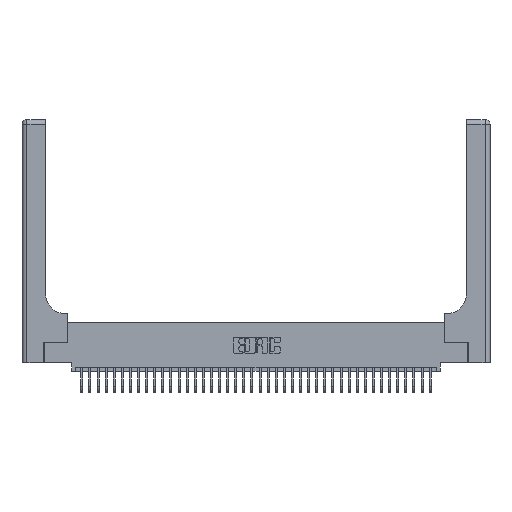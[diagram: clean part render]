
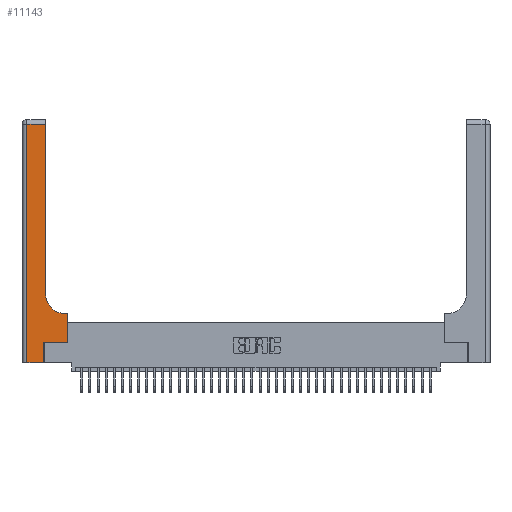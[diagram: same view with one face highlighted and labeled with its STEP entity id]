
A CAD part, top view. The second image highlights one B-rep face of the part: STEP entity #11143.
In plain terms, the highlighted planar face has unit normal (0, 0, 1).
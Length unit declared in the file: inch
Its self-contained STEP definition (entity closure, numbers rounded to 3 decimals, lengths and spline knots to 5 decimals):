
#72 = AXIS2_PLACEMENT_3D ( 'NONE', #17433, #11621, #32320 ) ;
#553 = CARTESIAN_POINT ( 'NONE',  ( 0.06, 0., 0.37 ) ) ;
#1645 = ORIENTED_EDGE ( 'NONE', *, *, #7474, .T. ) ;
#1949 = VECTOR ( 'NONE', #23740, 39.37008 ) ;
#2693 = CARTESIAN_POINT ( 'NONE',  ( 0.5585, 0.25, 0.37 ) ) ;
#3499 = ORIENTED_EDGE ( 'NONE', *, *, #9004, .T. ) ;
#3539 = VECTOR ( 'NONE', #17329, 39.37008 ) ;
#3942 = CARTESIAN_POINT ( 'NONE',  ( 0.5415, 0.6, 0.37 ) ) ;
#4141 = DIRECTION ( 'NONE',  ( -1., 0., 0. ) ) ;
#4835 = ORIENTED_EDGE ( 'NONE', *, *, #32792, .T. ) ;
#5052 = VERTEX_POINT ( 'NONE', #33338 ) ;
#5417 = VERTEX_POINT ( 'NONE', #2693 ) ;
#5472 = FACE_OUTER_BOUND ( 'NONE', #10474, .T. ) ;
#5539 = VECTOR ( 'NONE', #4141, 39.37008 ) ;
#6266 = EDGE_CURVE ( 'NONE', #5052, #35766, #32629, .T. ) ;
#6689 = LINE ( 'NONE', #22440, #13618 ) ;
#7474 = EDGE_CURVE ( 'NONE', #10615, #5417, #6689, .T. ) ;
#8162 = EDGE_CURVE ( 'NONE', #12874, #15630, #37588, .T. ) ;
#8182 = CARTESIAN_POINT ( 'NONE',  ( 0.2915, 2.94, 0.37 ) ) ;
#8233 = CARTESIAN_POINT ( 'NONE',  ( 0.2915, 0.6, 0.37 ) ) ;
#8654 = PLANE ( 'NONE',  #72 ) ;
#8872 = DIRECTION ( 'NONE',  ( 0., 0., -1. ) ) ;
#8981 = CARTESIAN_POINT ( 'NONE',  ( 0.269, 0., 0.37 ) ) ;
#9004 = EDGE_CURVE ( 'NONE', #10322, #10615, #33401, .T. ) ;
#9032 = ORIENTED_EDGE ( 'NONE', *, *, #26542, .T. ) ;
#9458 = CARTESIAN_POINT ( 'NONE',  ( 0.269, 0.25, 0.37 ) ) ;
#10322 = VERTEX_POINT ( 'NONE', #31474 ) ;
#10474 = EDGE_LOOP ( 'NONE', ( #24322, #20071, #26566, #4835, #3499, #1645, #9032, #14103, #28982 ) ) ;
#10615 = VERTEX_POINT ( 'NONE', #9458 ) ;
#11103 = AXIS2_PLACEMENT_3D ( 'NONE', #26612, #8872, #29576 ) ;
#11143 = ADVANCED_FACE ( 'NONE', ( #5472 ), #8654, .F. ) ;
#11621 = DIRECTION ( 'NONE',  ( 0., 0., -1. ) ) ;
#12874 = VERTEX_POINT ( 'NONE', #38023 ) ;
#13365 = LINE ( 'NONE', #8233, #14311 ) ;
#13618 = VECTOR ( 'NONE', #23081, 39.37008 ) ;
#13665 = CARTESIAN_POINT ( 'NONE',  ( 0.5585, 0.25, 0.37 ) ) ;
#14034 = VECTOR ( 'NONE', #34871, 39.37008 ) ;
#14103 = ORIENTED_EDGE ( 'NONE', *, *, #16040, .T. ) ;
#14195 = CARTESIAN_POINT ( 'NONE',  ( 0.06, 3., 0.37 ) ) ;
#14311 = VECTOR ( 'NONE', #28950, 39.37008 ) ;
#14358 = CARTESIAN_POINT ( 'NONE',  ( 0., 0., 0.37 ) ) ;
#15630 = VERTEX_POINT ( 'NONE', #553 ) ;
#16040 = EDGE_CURVE ( 'NONE', #32723, #28196, #13365, .T. ) ;
#17329 = DIRECTION ( 'NONE',  ( 1., 0., 0. ) ) ;
#17433 = CARTESIAN_POINT ( 'NONE',  ( 0., 3., 0.37 ) ) ;
#17809 = VECTOR ( 'NONE', #30040, 39.37008 ) ;
#18757 = CARTESIAN_POINT ( 'NONE',  ( 0.5585, 0.6, 0.37 ) ) ;
#19516 = DIRECTION ( 'NONE',  ( 0., 1., 0. ) ) ;
#20071 = ORIENTED_EDGE ( 'NONE', *, *, #30966, .T. ) ;
#22440 = CARTESIAN_POINT ( 'NONE',  ( 0.269, 0.25, 0.37 ) ) ;
#23081 = DIRECTION ( 'NONE',  ( 1., 0., 0. ) ) ;
#23740 = DIRECTION ( 'NONE',  ( 0., 1., 0. ) ) ;
#24322 = ORIENTED_EDGE ( 'NONE', *, *, #6266, .T. ) ;
#24854 = CARTESIAN_POINT ( 'NONE',  ( 0., 2.94, 0.37 ) ) ;
#26542 = EDGE_CURVE ( 'NONE', #5417, #32723, #31369, .T. ) ;
#26566 = ORIENTED_EDGE ( 'NONE', *, *, #8162, .T. ) ;
#26612 = CARTESIAN_POINT ( 'NONE',  ( 0.5415, 0.85, 0.37 ) ) ;
#27176 = LINE ( 'NONE', #14358, #3539 ) ;
#27324 = LINE ( 'NONE', #24854, #5539 ) ;
#28196 = VERTEX_POINT ( 'NONE', #3942 ) ;
#28504 = CIRCLE ( 'NONE', #11103, 0.25 ) ;
#28950 = DIRECTION ( 'NONE',  ( -1., 0., 0. ) ) ;
#28982 = ORIENTED_EDGE ( 'NONE', *, *, #33414, .T. ) ;
#29576 = DIRECTION ( 'NONE',  ( 1., 0., 0. ) ) ;
#30040 = DIRECTION ( 'NONE',  ( 0., 1., 0. ) ) ;
#30431 = VECTOR ( 'NONE', #19516, 39.37008 ) ;
#30966 = EDGE_CURVE ( 'NONE', #35766, #12874, #27324, .T. ) ;
#31369 = LINE ( 'NONE', #13665, #30431 ) ;
#31474 = CARTESIAN_POINT ( 'NONE',  ( 0.269, 0., 0.37 ) ) ;
#32320 = DIRECTION ( 'NONE',  ( -1., 0., 0. ) ) ;
#32629 = LINE ( 'NONE', #36066, #17809 ) ;
#32723 = VERTEX_POINT ( 'NONE', #18757 ) ;
#32792 = EDGE_CURVE ( 'NONE', #15630, #10322, #27176, .T. ) ;
#33338 = CARTESIAN_POINT ( 'NONE',  ( 0.2915, 0.85, 0.37 ) ) ;
#33401 = LINE ( 'NONE', #8981, #1949 ) ;
#33414 = EDGE_CURVE ( 'NONE', #28196, #5052, #28504, .T. ) ;
#34871 = DIRECTION ( 'NONE',  ( 0., -1., 0. ) ) ;
#35766 = VERTEX_POINT ( 'NONE', #8182 ) ;
#36066 = CARTESIAN_POINT ( 'NONE',  ( 0.2915, 3., 0.37 ) ) ;
#37588 = LINE ( 'NONE', #14195, #14034 ) ;
#38023 = CARTESIAN_POINT ( 'NONE',  ( 0.06, 2.94, 0.37 ) ) ;
